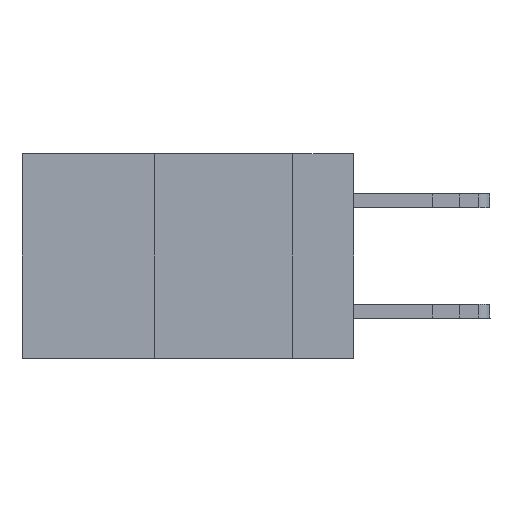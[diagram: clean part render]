
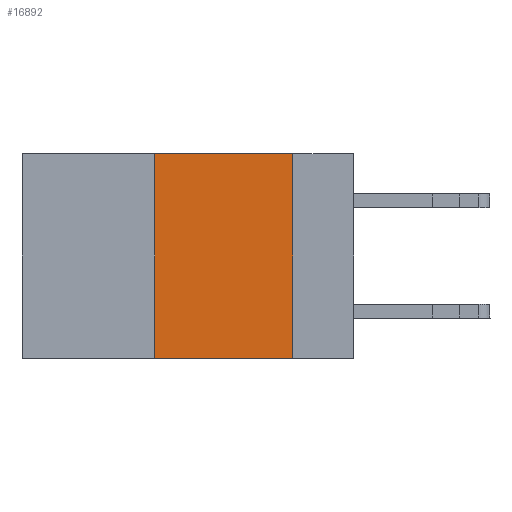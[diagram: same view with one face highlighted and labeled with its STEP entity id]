
A CAD part, left-side view. The second image highlights one B-rep face of the part: STEP entity #16892.
In plain terms, the highlighted planar face has unit normal (-1, 0, 0).
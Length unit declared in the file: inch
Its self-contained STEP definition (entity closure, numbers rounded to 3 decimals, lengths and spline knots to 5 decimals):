
#325 = FACE_OUTER_BOUND ( 'NONE', #8920, .T. ) ;
#357 = CARTESIAN_POINT ( 'NONE',  ( 0., 0.6, -0.37 ) ) ;
#550 = DIRECTION ( 'NONE',  ( 0., -1., 0. ) ) ;
#837 = PLANE ( 'NONE',  #15450 ) ;
#1849 = EDGE_CURVE ( 'NONE', #12034, #2878, #19320, .T. ) ;
#2163 = CARTESIAN_POINT ( 'NONE',  ( 0., 0.6, 0. ) ) ;
#2232 = VECTOR ( 'NONE', #15202, 39.37008 ) ;
#2782 = LINE ( 'NONE', #13487, #2232 ) ;
#2878 = VERTEX_POINT ( 'NONE', #11477 ) ;
#5299 = EDGE_CURVE ( 'NONE', #17010, #9843, #19424, .T. ) ;
#5429 = DIRECTION ( 'NONE',  ( 0., -1., 0. ) ) ;
#6197 = CARTESIAN_POINT ( 'NONE',  ( 0., 0.36, 0. ) ) ;
#6360 = CARTESIAN_POINT ( 'NONE',  ( 0., 0.6, 0. ) ) ;
#6385 = EDGE_CURVE ( 'NONE', #9843, #2878, #2782, .T. ) ;
#6393 = ORIENTED_EDGE ( 'NONE', *, *, #7962, .F. ) ;
#6965 = CARTESIAN_POINT ( 'NONE',  ( 0., 0.36, -0.37 ) ) ;
#7046 = VECTOR ( 'NONE', #14792, 39.37008 ) ;
#7497 = ORIENTED_EDGE ( 'NONE', *, *, #1849, .T. ) ;
#7962 = EDGE_CURVE ( 'NONE', #12034, #17010, #20065, .T. ) ;
#8081 = DIRECTION ( 'NONE',  ( 0., 0., -1. ) ) ;
#8920 = EDGE_LOOP ( 'NONE', ( #21469, #9284, #6393, #7497 ) ) ;
#9284 = ORIENTED_EDGE ( 'NONE', *, *, #5299, .F. ) ;
#9840 = CARTESIAN_POINT ( 'NONE',  ( 0., 0.11, 0. ) ) ;
#9843 = VERTEX_POINT ( 'NONE', #9840 ) ;
#10389 = VECTOR ( 'NONE', #550, 39.37008 ) ;
#11477 = CARTESIAN_POINT ( 'NONE',  ( 0., 0.11, -0.37 ) ) ;
#12034 = VERTEX_POINT ( 'NONE', #6965 ) ;
#13487 = CARTESIAN_POINT ( 'NONE',  ( 0., 0.11, 0. ) ) ;
#14792 = DIRECTION ( 'NONE',  ( 0., 0., 1. ) ) ;
#14900 = VECTOR ( 'NONE', #5429, 39.37008 ) ;
#15202 = DIRECTION ( 'NONE',  ( 0., 0., -1. ) ) ;
#15450 = AXIS2_PLACEMENT_3D ( 'NONE', #6360, #18286, #8081 ) ;
#16892 = ADVANCED_FACE ( 'NONE', ( #325 ), #837, .F. ) ;
#16962 = CARTESIAN_POINT ( 'NONE',  ( 0., 0.36, 0. ) ) ;
#17010 = VERTEX_POINT ( 'NONE', #16962 ) ;
#18286 = DIRECTION ( 'NONE',  ( 1., 0., 0. ) ) ;
#19320 = LINE ( 'NONE', #357, #14900 ) ;
#19424 = LINE ( 'NONE', #2163, #10389 ) ;
#20065 = LINE ( 'NONE', #6197, #7046 ) ;
#21469 = ORIENTED_EDGE ( 'NONE', *, *, #6385, .F. ) ;
